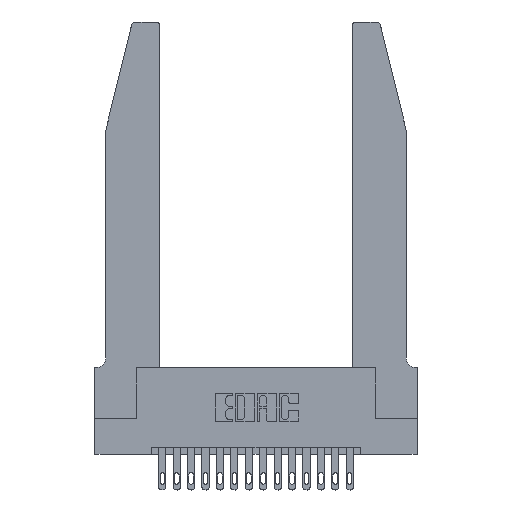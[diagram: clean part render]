
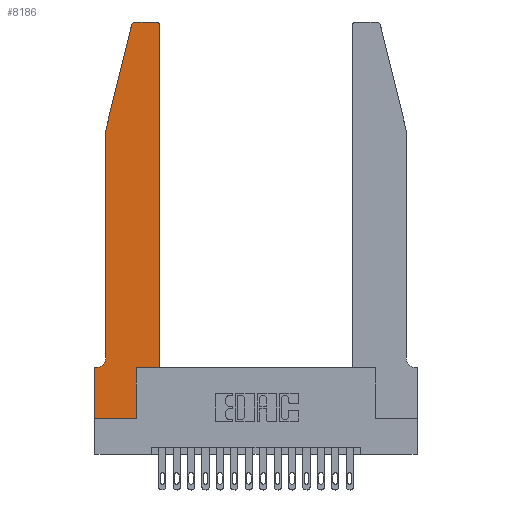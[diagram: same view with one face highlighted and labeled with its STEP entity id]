
A CAD part, top view. The second image highlights one B-rep face of the part: STEP entity #8186.
In plain terms, the highlighted planar face has unit normal (0, 0, 1).
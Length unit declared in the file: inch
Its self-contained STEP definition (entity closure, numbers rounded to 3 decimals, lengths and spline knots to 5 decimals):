
#202 = DIRECTION ( 'NONE',  ( 0., -1., 0. ) ) ;
#262 = EDGE_CURVE ( 'NONE', #1259, #5041, #18382, .T. ) ;
#298 = CARTESIAN_POINT ( 'NONE',  ( 0.284, 2.72, 0.37 ) ) ;
#693 = DIRECTION ( 'NONE',  ( -1., 0., 0. ) ) ;
#783 = CARTESIAN_POINT ( 'NONE',  ( 0.2865, 0., 0.37 ) ) ;
#1092 = CARTESIAN_POINT ( 'NONE',  ( 0.4505, 0.35, 0.37 ) ) ;
#1103 = CARTESIAN_POINT ( 'NONE',  ( 0.0755, 0.35, 0.37 ) ) ;
#1259 = VERTEX_POINT ( 'NONE', #5133 ) ;
#1260 = AXIS2_PLACEMENT_3D ( 'NONE', #4415, #12040, #4486 ) ;
#1323 = VERTEX_POINT ( 'NONE', #12775 ) ;
#1477 = VERTEX_POINT ( 'NONE', #13339 ) ;
#1611 = VERTEX_POINT ( 'NONE', #4731 ) ;
#1674 = VERTEX_POINT ( 'NONE', #12420 ) ;
#1710 = CARTESIAN_POINT ( 'NONE',  ( 0.0055, 0.42, 0.37 ) ) ;
#1747 = PLANE ( 'NONE',  #10818 ) ;
#1949 = EDGE_CURVE ( 'NONE', #7655, #14510, #3317, .T. ) ;
#2018 = DIRECTION ( 'NONE',  ( 0., 0., 1. ) ) ;
#2340 = LINE ( 'NONE', #14630, #15716 ) ;
#2674 = DIRECTION ( 'NONE',  ( 0., 1., 0. ) ) ;
#2781 = EDGE_CURVE ( 'NONE', #1477, #1259, #7270, .T. ) ;
#3197 = VECTOR ( 'NONE', #8193, 39.37008 ) ;
#3317 = LINE ( 'NONE', #1092, #5663 ) ;
#3388 = DIRECTION ( 'NONE',  ( 0., 0., -1. ) ) ;
#3712 = DIRECTION ( 'NONE',  ( 0., 1., 0. ) ) ;
#3720 = ORIENTED_EDGE ( 'NONE', *, *, #262, .T. ) ;
#3894 = CARTESIAN_POINT ( 'NONE',  ( 0.2865, 0.35, 0.37 ) ) ;
#4415 = CARTESIAN_POINT ( 'NONE',  ( 0.4205, 2.72, 0.37 ) ) ;
#4486 = DIRECTION ( 'NONE',  ( 1., 0., 0. ) ) ;
#4731 = CARTESIAN_POINT ( 'NONE',  ( 0.0755, 2., 0.37 ) ) ;
#4981 = LINE ( 'NONE', #7156, #6404 ) ;
#5030 = CARTESIAN_POINT ( 'NONE',  ( 0.4505, 2.72, 0.37 ) ) ;
#5041 = VERTEX_POINT ( 'NONE', #16720 ) ;
#5087 = LINE ( 'NONE', #13019, #3197 ) ;
#5133 = CARTESIAN_POINT ( 'NONE',  ( 0.284, 2.75, 0.37 ) ) ;
#5658 = CIRCLE ( 'NONE', #1260, 0.03 ) ;
#5663 = VECTOR ( 'NONE', #10110, 39.37008 ) ;
#6306 = EDGE_CURVE ( 'NONE', #16028, #7655, #7359, .T. ) ;
#6404 = VECTOR ( 'NONE', #11698, 39.37008 ) ;
#6622 = ORIENTED_EDGE ( 'NONE', *, *, #18196, .T. ) ;
#7156 = CARTESIAN_POINT ( 'NONE',  ( 0.0755, 2., 0.37 ) ) ;
#7270 = LINE ( 'NONE', #14957, #14568 ) ;
#7359 = LINE ( 'NONE', #3894, #16269 ) ;
#7377 = ORIENTED_EDGE ( 'NONE', *, *, #11483, .T. ) ;
#7410 = EDGE_CURVE ( 'NONE', #1323, #12525, #12985, .T. ) ;
#7520 = VECTOR ( 'NONE', #202, 39.37008 ) ;
#7595 = EDGE_LOOP ( 'NONE', ( #12995, #3720, #15297, #15403, #10198, #6622, #14575, #7377, #9865, #14814, #13978, #16546 ) ) ;
#7655 = VERTEX_POINT ( 'NONE', #17567 ) ;
#8186 = ADVANCED_FACE ( 'NONE', ( #12478 ), #1747, .T. ) ;
#8193 = DIRECTION ( 'NONE',  ( 1., 0., 0. ) ) ;
#8407 = VERTEX_POINT ( 'NONE', #11509 ) ;
#8453 = LINE ( 'NONE', #1103, #13872 ) ;
#8874 = EDGE_CURVE ( 'NONE', #18231, #1477, #5658, .T. ) ;
#8923 = EDGE_CURVE ( 'NONE', #1674, #8407, #17876, .T. ) ;
#9585 = EDGE_CURVE ( 'NONE', #14510, #18231, #2340, .T. ) ;
#9865 = ORIENTED_EDGE ( 'NONE', *, *, #6306, .T. ) ;
#10110 = DIRECTION ( 'NONE',  ( 1., 0., 0. ) ) ;
#10198 = ORIENTED_EDGE ( 'NONE', *, *, #7410, .T. ) ;
#10818 = AXIS2_PLACEMENT_3D ( 'NONE', #16899, #18269, #17554 ) ;
#11095 = VECTOR ( 'NONE', #11431, 39.37008 ) ;
#11431 = DIRECTION ( 'NONE',  ( 0., -1., 0. ) ) ;
#11483 = EDGE_CURVE ( 'NONE', #8407, #16028, #5087, .T. ) ;
#11509 = CARTESIAN_POINT ( 'NONE',  ( 0., 0., 0.37 ) ) ;
#11698 = DIRECTION ( 'NONE',  ( -0.239, -0.971, 0. ) ) ;
#11887 = DIRECTION ( 'NONE',  ( -1., 0., 0. ) ) ;
#11997 = AXIS2_PLACEMENT_3D ( 'NONE', #298, #2018, #13968 ) ;
#12040 = DIRECTION ( 'NONE',  ( 0., 0., 1. ) ) ;
#12420 = CARTESIAN_POINT ( 'NONE',  ( 0., 0.35, 0.37 ) ) ;
#12478 = FACE_OUTER_BOUND ( 'NONE', #7595, .T. ) ;
#12525 = VERTEX_POINT ( 'NONE', #18417 ) ;
#12775 = CARTESIAN_POINT ( 'NONE',  ( 0.0755, 0.42, 0.37 ) ) ;
#12904 = CARTESIAN_POINT ( 'NONE',  ( 0.0755, 2., 0.37 ) ) ;
#12985 = CIRCLE ( 'NONE', #16445, 0.07 ) ;
#12995 = ORIENTED_EDGE ( 'NONE', *, *, #2781, .T. ) ;
#13019 = CARTESIAN_POINT ( 'NONE',  ( 0., 0., 0.37 ) ) ;
#13339 = CARTESIAN_POINT ( 'NONE',  ( 0.4205, 2.75, 0.37 ) ) ;
#13782 = DIRECTION ( 'NONE',  ( -1., 0., 0. ) ) ;
#13872 = VECTOR ( 'NONE', #693, 39.37008 ) ;
#13968 = DIRECTION ( 'NONE',  ( 1., 0., 0. ) ) ;
#13978 = ORIENTED_EDGE ( 'NONE', *, *, #9585, .T. ) ;
#14510 = VERTEX_POINT ( 'NONE', #15435 ) ;
#14568 = VECTOR ( 'NONE', #11887, 39.37008 ) ;
#14575 = ORIENTED_EDGE ( 'NONE', *, *, #8923, .T. ) ;
#14630 = CARTESIAN_POINT ( 'NONE',  ( 0.4505, 0.35, 0.37 ) ) ;
#14814 = ORIENTED_EDGE ( 'NONE', *, *, #1949, .T. ) ;
#14957 = CARTESIAN_POINT ( 'NONE',  ( 0.2605, 2.75, 0.37 ) ) ;
#15044 = CARTESIAN_POINT ( 'NONE',  ( 0., 0., 0.37 ) ) ;
#15061 = LINE ( 'NONE', #12904, #11095 ) ;
#15297 = ORIENTED_EDGE ( 'NONE', *, *, #15804, .T. ) ;
#15403 = ORIENTED_EDGE ( 'NONE', *, *, #17055, .T. ) ;
#15435 = CARTESIAN_POINT ( 'NONE',  ( 0.4505, 0.35, 0.37 ) ) ;
#15716 = VECTOR ( 'NONE', #2674, 39.37008 ) ;
#15804 = EDGE_CURVE ( 'NONE', #5041, #1611, #4981, .T. ) ;
#16028 = VERTEX_POINT ( 'NONE', #783 ) ;
#16269 = VECTOR ( 'NONE', #3712, 39.37008 ) ;
#16445 = AXIS2_PLACEMENT_3D ( 'NONE', #1710, #3388, #13782 ) ;
#16546 = ORIENTED_EDGE ( 'NONE', *, *, #8874, .T. ) ;
#16720 = CARTESIAN_POINT ( 'NONE',  ( 0.25487, 2.72718, 0.37 ) ) ;
#16899 = CARTESIAN_POINT ( 'NONE',  ( 0., 0.35, 0.37 ) ) ;
#17055 = EDGE_CURVE ( 'NONE', #1611, #1323, #15061, .T. ) ;
#17554 = DIRECTION ( 'NONE',  ( 1., 0., 0. ) ) ;
#17567 = CARTESIAN_POINT ( 'NONE',  ( 0.2865, 0.35, 0.37 ) ) ;
#17876 = LINE ( 'NONE', #15044, #7520 ) ;
#18196 = EDGE_CURVE ( 'NONE', #12525, #1674, #8453, .T. ) ;
#18231 = VERTEX_POINT ( 'NONE', #5030 ) ;
#18269 = DIRECTION ( 'NONE',  ( 0., 0., 1. ) ) ;
#18382 = CIRCLE ( 'NONE', #11997, 0.03 ) ;
#18417 = CARTESIAN_POINT ( 'NONE',  ( 0.0055, 0.35, 0.37 ) ) ;
